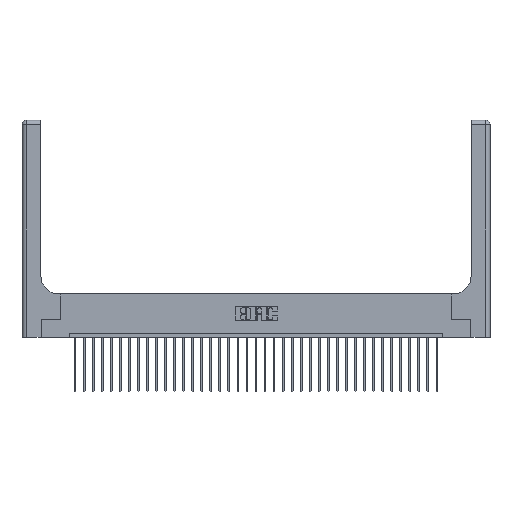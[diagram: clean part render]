
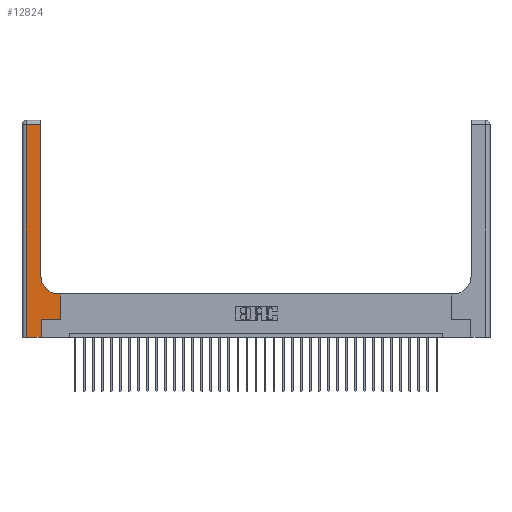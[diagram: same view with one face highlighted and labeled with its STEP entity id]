
A CAD part, top view. The second image highlights one B-rep face of the part: STEP entity #12824.
In plain terms, the highlighted planar face has unit normal (0, 0, 1).
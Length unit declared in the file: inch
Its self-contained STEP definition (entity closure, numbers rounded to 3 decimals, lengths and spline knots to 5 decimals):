
#480 = PLANE ( 'NONE',  #8444 ) ;
#972 = DIRECTION ( 'NONE',  ( 0., 1., 0. ) ) ;
#1187 = CARTESIAN_POINT ( 'NONE',  ( 0.51, 0.6, 0.37 ) ) ;
#1511 = ORIENTED_EDGE ( 'NONE', *, *, #9263, .T. ) ;
#1655 = DIRECTION ( 'NONE',  ( -1., 0., 0. ) ) ;
#1730 = EDGE_CURVE ( 'NONE', #27656, #3694, #17234, .T. ) ;
#2217 = LINE ( 'NONE', #31126, #17442 ) ;
#2395 = LINE ( 'NONE', #12030, #20678 ) ;
#2505 = EDGE_CURVE ( 'NONE', #17863, #27656, #4559, .T. ) ;
#2829 = DIRECTION ( 'NONE',  ( 0., 0., -1. ) ) ;
#2926 = DIRECTION ( 'NONE',  ( 1., 0., 0. ) ) ;
#3047 = CARTESIAN_POINT ( 'NONE',  ( 0.265, 0.25, 0.37 ) ) ;
#3378 = VECTOR ( 'NONE', #26422, 39.37008 ) ;
#3694 = VERTEX_POINT ( 'NONE', #20938 ) ;
#4420 = CARTESIAN_POINT ( 'NONE',  ( 0.06, 2.94, 0.37 ) ) ;
#4559 = LINE ( 'NONE', #19517, #21030 ) ;
#4984 = EDGE_CURVE ( 'NONE', #3694, #24541, #12948, .T. ) ;
#5385 = ORIENTED_EDGE ( 'NONE', *, *, #27341, .T. ) ;
#5455 = VECTOR ( 'NONE', #25238, 39.37008 ) ;
#5632 = ORIENTED_EDGE ( 'NONE', *, *, #4984, .T. ) ;
#5710 = ORIENTED_EDGE ( 'NONE', *, *, #28806, .T. ) ;
#5776 = EDGE_LOOP ( 'NONE', ( #18355, #21839, #23118, #12511, #5632, #5710, #1511, #5385, #13454 ) ) ;
#5810 = CARTESIAN_POINT ( 'NONE',  ( 0.528, 0.25, 0.37 ) ) ;
#6392 = CIRCLE ( 'NONE', #24030, 0.25 ) ;
#6544 = CARTESIAN_POINT ( 'NONE',  ( 0.26, 0.6, 0.37 ) ) ;
#7372 = VERTEX_POINT ( 'NONE', #14222 ) ;
#7408 = DIRECTION ( 'NONE',  ( -1., 0., 0. ) ) ;
#7629 = DIRECTION ( 'NONE',  ( 0., 0., -1. ) ) ;
#8444 = AXIS2_PLACEMENT_3D ( 'NONE', #14815, #2829, #7408 ) ;
#9052 = VERTEX_POINT ( 'NONE', #18755 ) ;
#9263 = EDGE_CURVE ( 'NONE', #26852, #15692, #2395, .T. ) ;
#9604 = DIRECTION ( 'NONE',  ( 0., -1., 0. ) ) ;
#9635 = DIRECTION ( 'NONE',  ( -1., 0., 0. ) ) ;
#9823 = CARTESIAN_POINT ( 'NONE',  ( 0.51, 0.85, 0.37 ) ) ;
#12030 = CARTESIAN_POINT ( 'NONE',  ( 0.528, 0.25, 0.37 ) ) ;
#12511 = ORIENTED_EDGE ( 'NONE', *, *, #1730, .T. ) ;
#12521 = CARTESIAN_POINT ( 'NONE',  ( 0., 0., 0.37 ) ) ;
#12559 = LINE ( 'NONE', #24087, #19841 ) ;
#12738 = VECTOR ( 'NONE', #1655, 39.37008 ) ;
#12789 = EDGE_CURVE ( 'NONE', #7372, #17863, #2217, .T. ) ;
#12824 = ADVANCED_FACE ( 'NONE', ( #26847 ), #480, .F. ) ;
#12948 = LINE ( 'NONE', #22585, #28257 ) ;
#13454 = ORIENTED_EDGE ( 'NONE', *, *, #24485, .T. ) ;
#14222 = CARTESIAN_POINT ( 'NONE',  ( 0.26, 2.94, 0.37 ) ) ;
#14815 = CARTESIAN_POINT ( 'NONE',  ( 0., 3., 0.37 ) ) ;
#15585 = CARTESIAN_POINT ( 'NONE',  ( 0.26, 3., 0.37 ) ) ;
#15692 = VERTEX_POINT ( 'NONE', #31106 ) ;
#16060 = EDGE_CURVE ( 'NONE', #9052, #7372, #25701, .T. ) ;
#17234 = LINE ( 'NONE', #12521, #3378 ) ;
#17442 = VECTOR ( 'NONE', #9635, 39.37008 ) ;
#17863 = VERTEX_POINT ( 'NONE', #4420 ) ;
#18355 = ORIENTED_EDGE ( 'NONE', *, *, #16060, .T. ) ;
#18755 = CARTESIAN_POINT ( 'NONE',  ( 0.26, 0.85, 0.37 ) ) ;
#19517 = CARTESIAN_POINT ( 'NONE',  ( 0.06, 3., 0.37 ) ) ;
#19841 = VECTOR ( 'NONE', #2926, 39.37008 ) ;
#20678 = VECTOR ( 'NONE', #28944, 39.37008 ) ;
#20938 = CARTESIAN_POINT ( 'NONE',  ( 0.265, 0., 0.37 ) ) ;
#21030 = VECTOR ( 'NONE', #9604, 39.37008 ) ;
#21839 = ORIENTED_EDGE ( 'NONE', *, *, #12789, .T. ) ;
#22299 = CARTESIAN_POINT ( 'NONE',  ( 0.06, 0., 0.37 ) ) ;
#22585 = CARTESIAN_POINT ( 'NONE',  ( 0.265, 0., 0.37 ) ) ;
#22803 = LINE ( 'NONE', #6544, #12738 ) ;
#23118 = ORIENTED_EDGE ( 'NONE', *, *, #2505, .T. ) ;
#24030 = AXIS2_PLACEMENT_3D ( 'NONE', #9823, #7629, #29113 ) ;
#24087 = CARTESIAN_POINT ( 'NONE',  ( 0.265, 0.25, 0.37 ) ) ;
#24199 = VERTEX_POINT ( 'NONE', #1187 ) ;
#24485 = EDGE_CURVE ( 'NONE', #24199, #9052, #6392, .T. ) ;
#24541 = VERTEX_POINT ( 'NONE', #3047 ) ;
#25238 = DIRECTION ( 'NONE',  ( 0., 1., 0. ) ) ;
#25701 = LINE ( 'NONE', #15585, #5455 ) ;
#26422 = DIRECTION ( 'NONE',  ( 1., 0., 0. ) ) ;
#26847 = FACE_OUTER_BOUND ( 'NONE', #5776, .T. ) ;
#26852 = VERTEX_POINT ( 'NONE', #5810 ) ;
#27341 = EDGE_CURVE ( 'NONE', #15692, #24199, #22803, .T. ) ;
#27656 = VERTEX_POINT ( 'NONE', #22299 ) ;
#28257 = VECTOR ( 'NONE', #972, 39.37008 ) ;
#28806 = EDGE_CURVE ( 'NONE', #24541, #26852, #12559, .T. ) ;
#28944 = DIRECTION ( 'NONE',  ( 0., 1., 0. ) ) ;
#29113 = DIRECTION ( 'NONE',  ( 1., 0., 0. ) ) ;
#31106 = CARTESIAN_POINT ( 'NONE',  ( 0.528, 0.6, 0.37 ) ) ;
#31126 = CARTESIAN_POINT ( 'NONE',  ( 0., 2.94, 0.37 ) ) ;
